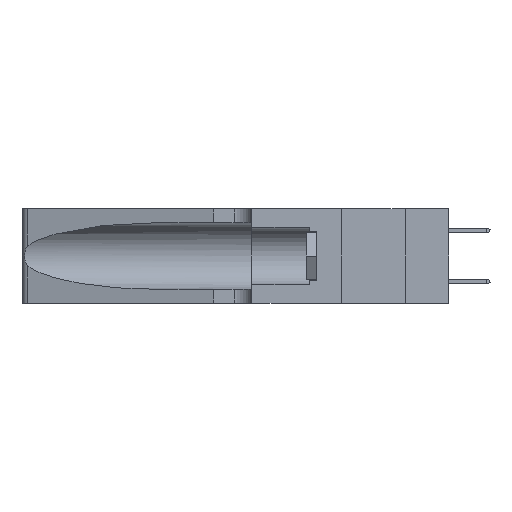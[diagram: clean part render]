
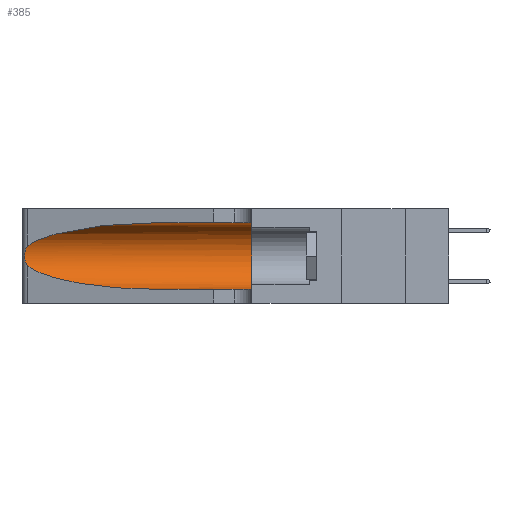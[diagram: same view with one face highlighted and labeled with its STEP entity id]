
A CAD part, left-side view. The second image highlights one B-rep face of the part: STEP entity #385.
In plain terms, the highlighted cylindrical face has radius 3.308 mm (diameter 6.617 mm), a partial arc.
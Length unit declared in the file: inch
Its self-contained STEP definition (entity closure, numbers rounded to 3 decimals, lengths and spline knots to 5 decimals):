
#385 = ADVANCED_FACE ( 'NONE', ( #12849 ), #5108, .F. ) ;
#792 = ORIENTED_EDGE ( 'NONE', *, *, #29337, .T. ) ;
#1577 = CARTESIAN_POINT ( 'NONE',  ( 0.25639, 1.23184, 0.21858 ) ) ;
#2113 = CARTESIAN_POINT ( 'NONE',  ( 0.1305, 1.61858, 0.05475 ) ) ;
#2252 = EDGE_CURVE ( 'NONE', #10263, #25006, #24662, .T. ) ;
#2591 = CARTESIAN_POINT ( 'NONE',  ( 0.1305, 0.72297, 0.05475 ) ) ;
#2779 = LINE ( 'NONE', #2113, #33504 ) ;
#3164 = CARTESIAN_POINT ( 'NONE',  ( 0.18966, 0.96281, 0.31525 ) ) ;
#4254 = CARTESIAN_POINT ( 'NONE',  ( 0.1305, 0.72297, 0.31525 ) ) ;
#4547 = EDGE_CURVE ( 'NONE', #5102, #9809, #2779, .T. ) ;
#5102 = VERTEX_POINT ( 'NONE', #29025 ) ;
#5108 = CYLINDRICAL_SURFACE ( 'NONE', #32848, 0.13025 ) ;
#5116 = CARTESIAN_POINT ( 'NONE',  ( 0.1305, 0.35, 0.31525 ) ) ;
#5430 = CARTESIAN_POINT ( 'NONE',  ( 0.1305, 0.72297, 0.31525 ) ) ;
#5542 = CIRCLE ( 'NONE', #22680, 0.13025 ) ;
#5595 = CARTESIAN_POINT ( 'NONE',  ( 0.1305, 0.35, 0.185 ) ) ;
#6256 = ORIENTED_EDGE ( 'NONE', *, *, #19842, .F. ) ;
#6789 = CARTESIAN_POINT ( 'NONE',  ( 0.26075, 1.23896, 0.178 ) ) ;
#7441 = CARTESIAN_POINT ( 'NONE',  ( 0.25487, 1.22718, 0.22369 ) ) ;
#7772 = EDGE_LOOP ( 'NONE', ( #33372, #792, #12511, #17688, #19138, #6256 ) ) ;
#9678 = CARTESIAN_POINT ( 'NONE',  ( 0.25555, 1.22994, 0.2215 ) ) ;
#9809 = VERTEX_POINT ( 'NONE', #30171 ) ;
#10263 = VERTEX_POINT ( 'NONE', #4254 ) ;
#10605 = LINE ( 'NONE', #23956, #11852 ) ;
#11336 = VERTEX_POINT ( 'NONE', #5116 ) ;
#11852 = VECTOR ( 'NONE', #29196, 39.37008 ) ;
#12309 = CARTESIAN_POINT ( 'NONE',  ( 0.25555, 1.22993, 0.14849 ) ) ;
#12428 = CARTESIAN_POINT ( 'NONE',  ( 0.25854, 1.2359, 0.20912 ) ) ;
#12511 = ORIENTED_EDGE ( 'NONE', *, *, #25960, .T. ) ;
#12849 = FACE_OUTER_BOUND ( 'NONE', #7772, .T. ) ;
#13334 = CARTESIAN_POINT ( 'NONE',  ( 0.18966, 0.96281, 0.05475 ) ) ;
#13843 = DIRECTION ( 'NONE',  ( 0., 1., 0. ) ) ;
#15051 = CARTESIAN_POINT ( 'NONE',  ( 0.25487, 1.22718, 0.14631 ) ) ;
#15991 = VERTEX_POINT ( 'NONE', #30024 ) ;
#16345 =( BOUNDED_CURVE ( )  B_SPLINE_CURVE ( 3, ( #31869, #34560, #13334, #2591 ),
 .UNSPECIFIED., .F., .F. ) 
 B_SPLINE_CURVE_WITH_KNOTS ( ( 4, 4 ),
 ( 3.44316, 4.71239 ),
 .UNSPECIFIED. ) 
 CURVE ( )  GEOMETRIC_REPRESENTATION_ITEM ( )  RATIONAL_B_SPLINE_CURVE ( ( 1., 0.87, 0.87, 1. ) ) 
 REPRESENTATION_ITEM ( '' )  );
#17688 = ORIENTED_EDGE ( 'NONE', *, *, #4547, .T. ) ;
#17736 = CARTESIAN_POINT ( 'NONE',  ( 0.26075, 1.23896, 0.19203 ) ) ;
#18083 = CARTESIAN_POINT ( 'NONE',  ( 0.26017, 1.23833, 0.17102 ) ) ;
#19138 = ORIENTED_EDGE ( 'NONE', *, *, #31813, .F. ) ;
#19842 = EDGE_CURVE ( 'NONE', #10263, #11336, #10605, .T. ) ;
#20526 = CARTESIAN_POINT ( 'NONE',  ( 0.1305, 1.61858, 0.185 ) ) ;
#20965 = CARTESIAN_POINT ( 'NONE',  ( 0.25787, 1.23484, 0.2124 ) ) ;
#21280 = DIRECTION ( 'NONE',  ( 0., -1., 0. ) ) ;
#21493 = DIRECTION ( 'NONE',  ( 0., 0., -1. ) ) ;
#22680 = AXIS2_PLACEMENT_3D ( 'NONE', #5595, #13843, #24846 ) ;
#22751 = DIRECTION ( 'NONE',  ( 0., -1., 0. ) ) ;
#23302 = CARTESIAN_POINT ( 'NONE',  ( 0.25487, 1.22718, 0.22369 ) ) ;
#23678 = CARTESIAN_POINT ( 'NONE',  ( 0.26018, 1.23835, 0.19895 ) ) ;
#23956 = CARTESIAN_POINT ( 'NONE',  ( 0.1305, 1.61858, 0.31525 ) ) ;
#24662 =( BOUNDED_CURVE ( )  B_SPLINE_CURVE ( 3, ( #5430, #3164, #30287, #30173 ),
 .UNSPECIFIED., .F., .T. ) 
 B_SPLINE_CURVE_WITH_KNOTS ( ( 4, 4 ),
 ( 1.5708, 2.84003 ),
 .UNSPECIFIED. ) 
 CURVE ( )  GEOMETRIC_REPRESENTATION_ITEM ( )  RATIONAL_B_SPLINE_CURVE ( ( 1., 0.87, 0.87, 1. ) ) 
 REPRESENTATION_ITEM ( '' )  );
#24846 = DIRECTION ( 'NONE',  ( 0., 0., 1. ) ) ;
#25006 = VERTEX_POINT ( 'NONE', #7441 ) ;
#25960 = EDGE_CURVE ( 'NONE', #15991, #5102, #16345, .T. ) ;
#28647 = CARTESIAN_POINT ( 'NONE',  ( 0.25639, 1.23186, 0.15144 ) ) ;
#29025 = CARTESIAN_POINT ( 'NONE',  ( 0.1305, 0.72297, 0.05475 ) ) ;
#29196 = DIRECTION ( 'NONE',  ( 0., -1., 0. ) ) ;
#29337 = EDGE_CURVE ( 'NONE', #25006, #15991, #32751, .T. ) ;
#30024 = CARTESIAN_POINT ( 'NONE',  ( 0.25487, 1.22718, 0.14631 ) ) ;
#30171 = CARTESIAN_POINT ( 'NONE',  ( 0.1305, 0.35, 0.05475 ) ) ;
#30173 = CARTESIAN_POINT ( 'NONE',  ( 0.25487, 1.22718, 0.22369 ) ) ;
#30287 = CARTESIAN_POINT ( 'NONE',  ( 0.2373, 1.15595, 0.28018 ) ) ;
#31547 = CARTESIAN_POINT ( 'NONE',  ( 0.25789, 1.23486, 0.15765 ) ) ;
#31813 = EDGE_CURVE ( 'NONE', #11336, #9809, #5542, .T. ) ;
#31869 = CARTESIAN_POINT ( 'NONE',  ( 0.25487, 1.22718, 0.14631 ) ) ;
#32751 = B_SPLINE_CURVE_WITH_KNOTS ( 'NONE', 3,
 ( #23302, #9678, #1577, #20965, #12428, #23678, #17736, #6789, #18083, #34141, #31547, #28647, #12309, #15051 ),
 .UNSPECIFIED., .F., .F.,
 ( 4, 2, 2, 2, 2, 2, 4 ),
 ( 0., 0.00027, 0.00053, 0.00107, 0.0016, 0.00187, 0.00214 ),
 .UNSPECIFIED. ) ;
#32848 = AXIS2_PLACEMENT_3D ( 'NONE', #20526, #22751, #21493 ) ;
#33372 = ORIENTED_EDGE ( 'NONE', *, *, #2252, .T. ) ;
#33504 = VECTOR ( 'NONE', #21280, 39.37008 ) ;
#34141 = CARTESIAN_POINT ( 'NONE',  ( 0.25856, 1.23593, 0.16098 ) ) ;
#34560 = CARTESIAN_POINT ( 'NONE',  ( 0.2373, 1.15595, 0.08982 ) ) ;
